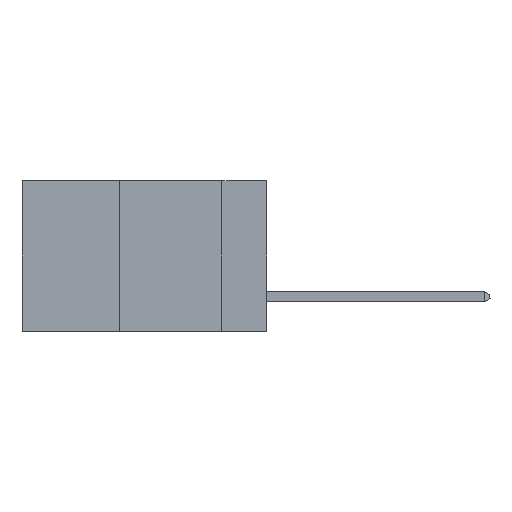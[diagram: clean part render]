
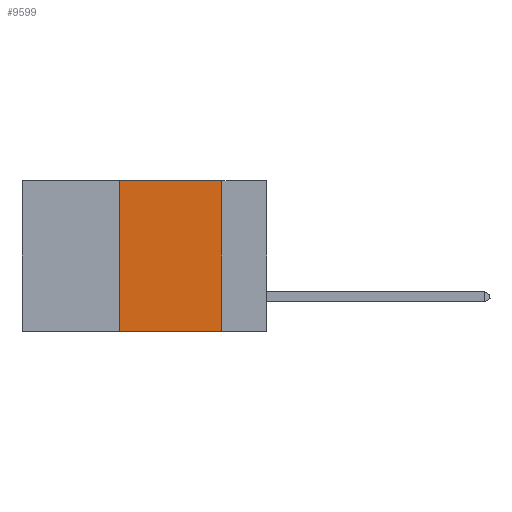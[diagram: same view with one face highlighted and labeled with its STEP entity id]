
A CAD part, left-side view. The second image highlights one B-rep face of the part: STEP entity #9599.
In plain terms, the highlighted planar face has unit normal (-1, 0, 0).
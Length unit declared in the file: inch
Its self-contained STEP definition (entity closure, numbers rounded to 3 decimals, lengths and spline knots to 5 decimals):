
#305 = VECTOR ( 'NONE', #16242, 39.37008 ) ;
#323 = VECTOR ( 'NONE', #8130, 39.37008 ) ;
#394 = CARTESIAN_POINT ( 'NONE',  ( 0., 0.36, 0. ) ) ;
#602 = AXIS2_PLACEMENT_3D ( 'NONE', #8264, #16225, #6728 ) ;
#2035 = PLANE ( 'NONE',  #602 ) ;
#2131 = FACE_OUTER_BOUND ( 'NONE', #15707, .T. ) ;
#2767 = ORIENTED_EDGE ( 'NONE', *, *, #18074, .F. ) ;
#4546 = CARTESIAN_POINT ( 'NONE',  ( 0., 0.11, 0. ) ) ;
#4641 = VERTEX_POINT ( 'NONE', #12954 ) ;
#4796 = ORIENTED_EDGE ( 'NONE', *, *, #15159, .F. ) ;
#6728 = DIRECTION ( 'NONE',  ( 0., 0., -1. ) ) ;
#6842 = CARTESIAN_POINT ( 'NONE',  ( 0., 0.6, -0.37 ) ) ;
#6876 = CARTESIAN_POINT ( 'NONE',  ( 0., 0.36, -0.37 ) ) ;
#8130 = DIRECTION ( 'NONE',  ( 0., -1., 0. ) ) ;
#8264 = CARTESIAN_POINT ( 'NONE',  ( 0., 0.6, 0. ) ) ;
#8414 = LINE ( 'NONE', #4546, #13864 ) ;
#9537 = LINE ( 'NONE', #6842, #323 ) ;
#9599 = ADVANCED_FACE ( 'NONE', ( #2131 ), #2035, .F. ) ;
#10479 = LINE ( 'NONE', #19548, #305 ) ;
#11469 = ORIENTED_EDGE ( 'NONE', *, *, #12045, .T. ) ;
#12045 = EDGE_CURVE ( 'NONE', #17238, #4641, #9537, .T. ) ;
#12919 = VECTOR ( 'NONE', #16507, 39.37008 ) ;
#12954 = CARTESIAN_POINT ( 'NONE',  ( 0., 0.11, -0.37 ) ) ;
#13071 = EDGE_CURVE ( 'NONE', #15396, #15390, #10479, .T. ) ;
#13133 = CARTESIAN_POINT ( 'NONE',  ( 0., 0.36, 0. ) ) ;
#13322 = CARTESIAN_POINT ( 'NONE',  ( 0., 0.11, 0. ) ) ;
#13864 = VECTOR ( 'NONE', #15677, 39.37008 ) ;
#15159 = EDGE_CURVE ( 'NONE', #15390, #4641, #8414, .T. ) ;
#15390 = VERTEX_POINT ( 'NONE', #13322 ) ;
#15396 = VERTEX_POINT ( 'NONE', #394 ) ;
#15677 = DIRECTION ( 'NONE',  ( 0., 0., -1. ) ) ;
#15707 = EDGE_LOOP ( 'NONE', ( #4796, #17760, #2767, #11469 ) ) ;
#16225 = DIRECTION ( 'NONE',  ( 1., 0., 0. ) ) ;
#16242 = DIRECTION ( 'NONE',  ( 0., -1., 0. ) ) ;
#16507 = DIRECTION ( 'NONE',  ( 0., 0., 1. ) ) ;
#17135 = LINE ( 'NONE', #13133, #12919 ) ;
#17238 = VERTEX_POINT ( 'NONE', #6876 ) ;
#17760 = ORIENTED_EDGE ( 'NONE', *, *, #13071, .F. ) ;
#18074 = EDGE_CURVE ( 'NONE', #17238, #15396, #17135, .T. ) ;
#19548 = CARTESIAN_POINT ( 'NONE',  ( 0., 0.6, 0. ) ) ;
